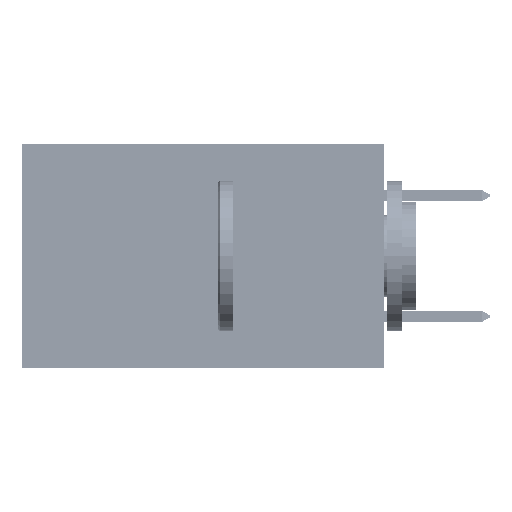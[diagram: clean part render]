
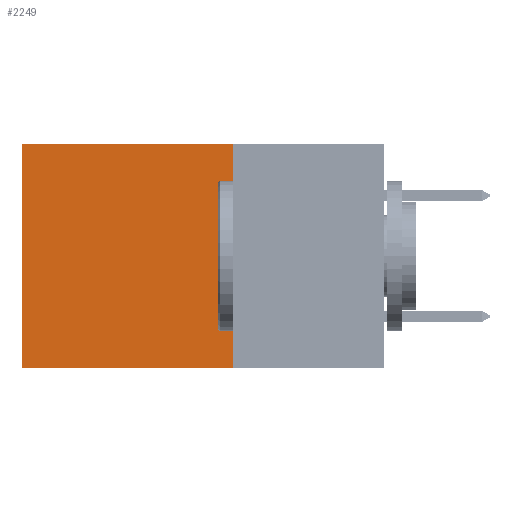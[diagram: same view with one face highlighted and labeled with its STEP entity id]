
A CAD part, left-side view. The second image highlights one B-rep face of the part: STEP entity #2249.
In plain terms, the highlighted planar face has unit normal (-1, 0, 0).
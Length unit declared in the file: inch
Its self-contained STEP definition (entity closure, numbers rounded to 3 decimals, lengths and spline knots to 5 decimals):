
#107 = LINE ( 'NONE', #4313, #9273 ) ;
#2249 = ADVANCED_FACE ( 'NONE', ( #4283 ), #11913, .F. ) ;
#2605 = VECTOR ( 'NONE', #41426, 39.37008 ) ;
#2727 = EDGE_CURVE ( 'NONE', #33750, #18885, #19588, .T. ) ;
#4283 = FACE_OUTER_BOUND ( 'NONE', #35244, .T. ) ;
#4313 = CARTESIAN_POINT ( 'NONE',  ( 0.2875, 0.25, -0.37 ) ) ;
#5667 = ORIENTED_EDGE ( 'NONE', *, *, #28646, .T. ) ;
#6762 = CARTESIAN_POINT ( 'NONE',  ( 0.2875, 0.25, 0. ) ) ;
#8820 = CARTESIAN_POINT ( 'NONE',  ( 0.2875, 0.25, -0.37 ) ) ;
#9273 = VECTOR ( 'NONE', #42748, 39.37008 ) ;
#11913 = PLANE ( 'NONE',  #25357 ) ;
#12563 = CARTESIAN_POINT ( 'NONE',  ( 0.2875, 0.25, 0. ) ) ;
#15207 = EDGE_CURVE ( 'NONE', #28846, #16077, #45874, .T. ) ;
#15847 = DIRECTION ( 'NONE',  ( 0., 0., -1. ) ) ;
#16077 = VERTEX_POINT ( 'NONE', #8820 ) ;
#18492 = DIRECTION ( 'NONE',  ( 0., 0., -1. ) ) ;
#18885 = VERTEX_POINT ( 'NONE', #39339 ) ;
#19559 = CARTESIAN_POINT ( 'NONE',  ( 0.2875, 0.25, 0. ) ) ;
#19588 = LINE ( 'NONE', #34042, #49005 ) ;
#21686 = ORIENTED_EDGE ( 'NONE', *, *, #35012, .F. ) ;
#24498 = CARTESIAN_POINT ( 'NONE',  ( 0.2875, 0.6, 0. ) ) ;
#25258 = DIRECTION ( 'NONE',  ( 0., 0., -1. ) ) ;
#25357 = AXIS2_PLACEMENT_3D ( 'NONE', #19559, #38959, #15847 ) ;
#28646 = EDGE_CURVE ( 'NONE', #28846, #33750, #46188, .T. ) ;
#28846 = VERTEX_POINT ( 'NONE', #12563 ) ;
#32197 = ORIENTED_EDGE ( 'NONE', *, *, #15207, .F. ) ;
#33750 = VERTEX_POINT ( 'NONE', #24498 ) ;
#34042 = CARTESIAN_POINT ( 'NONE',  ( 0.2875, 0.6, 0. ) ) ;
#35012 = EDGE_CURVE ( 'NONE', #16077, #18885, #107, .T. ) ;
#35244 = EDGE_LOOP ( 'NONE', ( #49512, #21686, #32197, #5667 ) ) ;
#35737 = VECTOR ( 'NONE', #25258, 39.37008 ) ;
#38959 = DIRECTION ( 'NONE',  ( 1., 0., 0. ) ) ;
#39339 = CARTESIAN_POINT ( 'NONE',  ( 0.2875, 0.6, -0.37 ) ) ;
#41426 = DIRECTION ( 'NONE',  ( 0., 1., 0. ) ) ;
#42748 = DIRECTION ( 'NONE',  ( 0., 1., 0. ) ) ;
#44411 = CARTESIAN_POINT ( 'NONE',  ( 0.2875, 0.25, 0. ) ) ;
#45874 = LINE ( 'NONE', #44411, #35737 ) ;
#46188 = LINE ( 'NONE', #6762, #2605 ) ;
#49005 = VECTOR ( 'NONE', #18492, 39.37008 ) ;
#49512 = ORIENTED_EDGE ( 'NONE', *, *, #2727, .T. ) ;
